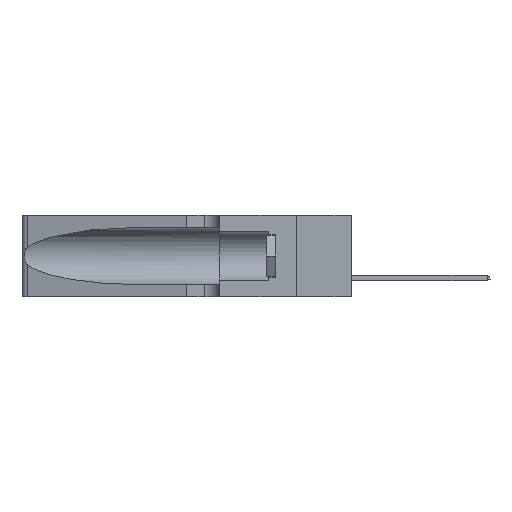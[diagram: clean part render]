
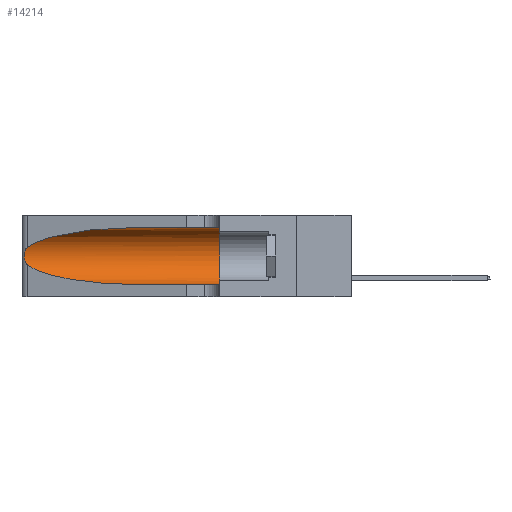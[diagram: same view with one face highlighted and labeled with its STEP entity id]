
A CAD part, left-side view. The second image highlights one B-rep face of the part: STEP entity #14214.
In plain terms, the highlighted cylindrical face has radius 3.308 mm (diameter 6.617 mm), a partial arc.
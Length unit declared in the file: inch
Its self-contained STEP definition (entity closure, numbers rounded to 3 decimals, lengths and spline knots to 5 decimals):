
#118 = EDGE_CURVE ( 'NONE', #17894, #2205, #12227, .T. ) ;
#140 = CARTESIAN_POINT ( 'NONE',  ( 0.1305, 0.35, 0.05475 ) ) ;
#603 = LINE ( 'NONE', #14160, #26928 ) ;
#1286 = CARTESIAN_POINT ( 'NONE',  ( 0.25555, 1.22994, 0.2215 ) ) ;
#1414 =( BOUNDED_CURVE ( )  B_SPLINE_CURVE ( 3, ( #12684, #10724, #10911, #27625 ),
 .UNSPECIFIED., .F., .F. ) 
 B_SPLINE_CURVE_WITH_KNOTS ( ( 4, 4 ),
 ( 3.44316, 4.71239 ),
 .UNSPECIFIED. ) 
 CURVE ( )  GEOMETRIC_REPRESENTATION_ITEM ( )  RATIONAL_B_SPLINE_CURVE ( ( 1., 0.87, 0.87, 1. ) ) 
 REPRESENTATION_ITEM ( '' )  );
#1559 = CARTESIAN_POINT ( 'NONE',  ( 0.25789, 1.23486, 0.15765 ) ) ;
#1920 = CARTESIAN_POINT ( 'NONE',  ( 0.26018, 1.23835, 0.19895 ) ) ;
#2205 = VERTEX_POINT ( 'NONE', #140 ) ;
#3560 = DIRECTION ( 'NONE',  ( 0., -1., 0. ) ) ;
#3802 = VERTEX_POINT ( 'NONE', #19863 ) ;
#3868 = CARTESIAN_POINT ( 'NONE',  ( 0.26075, 1.23896, 0.19203 ) ) ;
#4342 = ORIENTED_EDGE ( 'NONE', *, *, #118, .F. ) ;
#5516 = DIRECTION ( 'NONE',  ( 0., 0., 1. ) ) ;
#5660 = B_SPLINE_CURVE_WITH_KNOTS ( 'NONE', 3,
 ( #18489, #1286, #27204, #8249, #6194, #1920, #3868, #16692, #25312, #18578, #1559, #16415, #10289, #12442 ),
 .UNSPECIFIED., .F., .F.,
 ( 4, 2, 2, 2, 2, 2, 4 ),
 ( 0., 0.00027, 0.00053, 0.00107, 0.0016, 0.00187, 0.00214 ),
 .UNSPECIFIED. ) ;
#5938 = CARTESIAN_POINT ( 'NONE',  ( 0.1305, 0.72297, 0.31525 ) ) ;
#6194 = CARTESIAN_POINT ( 'NONE',  ( 0.25854, 1.2359, 0.20912 ) ) ;
#6321 = CARTESIAN_POINT ( 'NONE',  ( 0.18966, 0.96281, 0.31525 ) ) ;
#6905 = ORIENTED_EDGE ( 'NONE', *, *, #7069, .T. ) ;
#6941 = CARTESIAN_POINT ( 'NONE',  ( 0.25487, 1.22718, 0.14631 ) ) ;
#6992 = LINE ( 'NONE', #10645, #25035 ) ;
#7069 = EDGE_CURVE ( 'NONE', #17609, #7568, #1414, .T. ) ;
#7568 = VERTEX_POINT ( 'NONE', #11151 ) ;
#8249 = CARTESIAN_POINT ( 'NONE',  ( 0.25787, 1.23484, 0.2124 ) ) ;
#8600 = CARTESIAN_POINT ( 'NONE',  ( 0.1305, 1.61858, 0.185 ) ) ;
#10069 = CARTESIAN_POINT ( 'NONE',  ( 0.1305, 0.35, 0.185 ) ) ;
#10289 = CARTESIAN_POINT ( 'NONE',  ( 0.25555, 1.22993, 0.14849 ) ) ;
#10334 = CARTESIAN_POINT ( 'NONE',  ( 0.25487, 1.22718, 0.22369 ) ) ;
#10528 = ORIENTED_EDGE ( 'NONE', *, *, #13098, .F. ) ;
#10645 = CARTESIAN_POINT ( 'NONE',  ( 0.1305, 1.61858, 0.05475 ) ) ;
#10724 = CARTESIAN_POINT ( 'NONE',  ( 0.2373, 1.15595, 0.08982 ) ) ;
#10911 = CARTESIAN_POINT ( 'NONE',  ( 0.18966, 0.96281, 0.05475 ) ) ;
#11151 = CARTESIAN_POINT ( 'NONE',  ( 0.1305, 0.72297, 0.05475 ) ) ;
#11355 = EDGE_CURVE ( 'NONE', #17387, #3802, #12658, .T. ) ;
#12218 = DIRECTION ( 'NONE',  ( 0., 1., 0. ) ) ;
#12227 = CIRCLE ( 'NONE', #22099, 0.13025 ) ;
#12442 = CARTESIAN_POINT ( 'NONE',  ( 0.25487, 1.22718, 0.14631 ) ) ;
#12658 =( BOUNDED_CURVE ( )  B_SPLINE_CURVE ( 3, ( #25453, #6321, #23394, #10334 ),
 .UNSPECIFIED., .F., .F. ) 
 B_SPLINE_CURVE_WITH_KNOTS ( ( 4, 4 ),
 ( 1.5708, 2.84003 ),
 .UNSPECIFIED. ) 
 CURVE ( )  GEOMETRIC_REPRESENTATION_ITEM ( )  RATIONAL_B_SPLINE_CURVE ( ( 1., 0.87, 0.87, 1. ) ) 
 REPRESENTATION_ITEM ( '' )  );
#12684 = CARTESIAN_POINT ( 'NONE',  ( 0.25487, 1.22718, 0.14631 ) ) ;
#12701 = DIRECTION ( 'NONE',  ( 0., -1., 0. ) ) ;
#12922 = ORIENTED_EDGE ( 'NONE', *, *, #11355, .T. ) ;
#13098 = EDGE_CURVE ( 'NONE', #17387, #17894, #603, .T. ) ;
#14160 = CARTESIAN_POINT ( 'NONE',  ( 0.1305, 1.61858, 0.31525 ) ) ;
#14214 = ADVANCED_FACE ( 'NONE', ( #18135 ), #23513, .F. ) ;
#15197 = DIRECTION ( 'NONE',  ( 0., -1., 0. ) ) ;
#15842 = AXIS2_PLACEMENT_3D ( 'NONE', #8600, #15197, #25687 ) ;
#16415 = CARTESIAN_POINT ( 'NONE',  ( 0.25639, 1.23186, 0.15144 ) ) ;
#16675 = CARTESIAN_POINT ( 'NONE',  ( 0.1305, 0.35, 0.31525 ) ) ;
#16692 = CARTESIAN_POINT ( 'NONE',  ( 0.26075, 1.23896, 0.178 ) ) ;
#17387 = VERTEX_POINT ( 'NONE', #5938 ) ;
#17609 = VERTEX_POINT ( 'NONE', #6941 ) ;
#17894 = VERTEX_POINT ( 'NONE', #16675 ) ;
#17902 = EDGE_LOOP ( 'NONE', ( #12922, #27244, #6905, #20469, #4342, #10528 ) ) ;
#18135 = FACE_OUTER_BOUND ( 'NONE', #17902, .T. ) ;
#18489 = CARTESIAN_POINT ( 'NONE',  ( 0.25487, 1.22718, 0.22369 ) ) ;
#18578 = CARTESIAN_POINT ( 'NONE',  ( 0.25856, 1.23593, 0.16098 ) ) ;
#19863 = CARTESIAN_POINT ( 'NONE',  ( 0.25487, 1.22718, 0.22369 ) ) ;
#20246 = EDGE_CURVE ( 'NONE', #3802, #17609, #5660, .T. ) ;
#20469 = ORIENTED_EDGE ( 'NONE', *, *, #27441, .T. ) ;
#22099 = AXIS2_PLACEMENT_3D ( 'NONE', #10069, #12218, #5516 ) ;
#23394 = CARTESIAN_POINT ( 'NONE',  ( 0.2373, 1.15595, 0.28018 ) ) ;
#23513 = CYLINDRICAL_SURFACE ( 'NONE', #15842, 0.13025 ) ;
#25035 = VECTOR ( 'NONE', #12701, 39.37008 ) ;
#25312 = CARTESIAN_POINT ( 'NONE',  ( 0.26017, 1.23833, 0.17102 ) ) ;
#25453 = CARTESIAN_POINT ( 'NONE',  ( 0.1305, 0.72297, 0.31525 ) ) ;
#25687 = DIRECTION ( 'NONE',  ( 0., 0., -1. ) ) ;
#26928 = VECTOR ( 'NONE', #3560, 39.37008 ) ;
#27204 = CARTESIAN_POINT ( 'NONE',  ( 0.25639, 1.23184, 0.21858 ) ) ;
#27244 = ORIENTED_EDGE ( 'NONE', *, *, #20246, .T. ) ;
#27441 = EDGE_CURVE ( 'NONE', #7568, #2205, #6992, .T. ) ;
#27625 = CARTESIAN_POINT ( 'NONE',  ( 0.1305, 0.72297, 0.05475 ) ) ;
